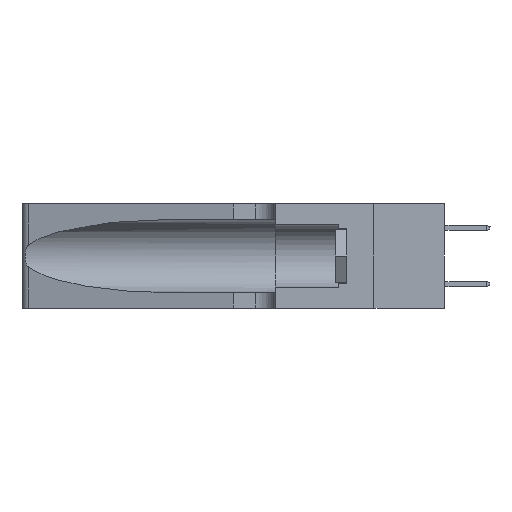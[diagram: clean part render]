
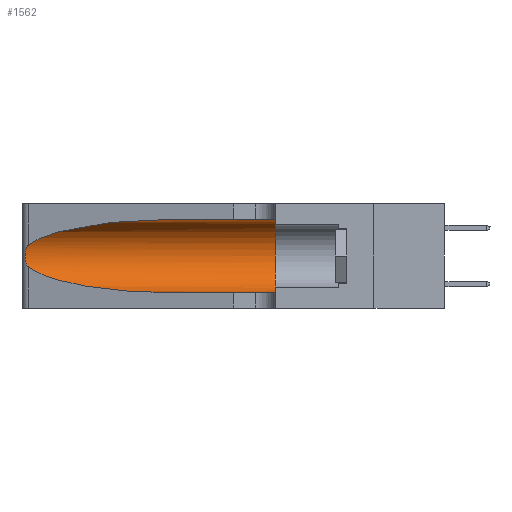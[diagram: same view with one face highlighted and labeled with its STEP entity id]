
A CAD part, left-side view. The second image highlights one B-rep face of the part: STEP entity #1562.
In plain terms, the highlighted cylindrical face has radius 3.308 mm (diameter 6.617 mm), a partial arc.
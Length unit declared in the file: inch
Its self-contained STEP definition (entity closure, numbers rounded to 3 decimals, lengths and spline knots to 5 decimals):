
#777 = CARTESIAN_POINT ( 'NONE',  ( 0.1305, 0.35, 0.05475 ) ) ;
#1447 = VERTEX_POINT ( 'NONE', #21464 ) ;
#1562 = ADVANCED_FACE ( 'NONE', ( #16014 ), #16576, .F. ) ;
#1746 = CARTESIAN_POINT ( 'NONE',  ( 0.25555, 1.22993, 0.14849 ) ) ;
#1816 = CARTESIAN_POINT ( 'NONE',  ( 0.25555, 1.22994, 0.2215 ) ) ;
#1904 = CARTESIAN_POINT ( 'NONE',  ( 0.1305, 0.72297, 0.31525 ) ) ;
#1925 =( BOUNDED_CURVE ( )  B_SPLINE_CURVE ( 3, ( #1904, #7684, #22179, #14631 ),
 .UNSPECIFIED., .F., .T. ) 
 B_SPLINE_CURVE_WITH_KNOTS ( ( 4, 4 ),
 ( 1.5708, 2.84003 ),
 .UNSPECIFIED. ) 
 CURVE ( )  GEOMETRIC_REPRESENTATION_ITEM ( )  RATIONAL_B_SPLINE_CURVE ( ( 1., 0.87, 0.87, 1. ) ) 
 REPRESENTATION_ITEM ( '' )  );
#1974 = CARTESIAN_POINT ( 'NONE',  ( 0.25639, 1.23186, 0.15144 ) ) ;
#1976 = DIRECTION ( 'NONE',  ( 0., -1., 0. ) ) ;
#2594 = VECTOR ( 'NONE', #1976, 39.37008 ) ;
#2981 = EDGE_CURVE ( 'NONE', #1447, #3437, #1925, .T. ) ;
#3400 =( BOUNDED_CURVE ( )  B_SPLINE_CURVE ( 3, ( #15521, #17353, #19363, #17596 ),
 .UNSPECIFIED., .F., .F. ) 
 B_SPLINE_CURVE_WITH_KNOTS ( ( 4, 4 ),
 ( 3.44316, 4.71239 ),
 .UNSPECIFIED. ) 
 CURVE ( )  GEOMETRIC_REPRESENTATION_ITEM ( )  RATIONAL_B_SPLINE_CURVE ( ( 1., 0.87, 0.87, 1. ) ) 
 REPRESENTATION_ITEM ( '' )  );
#3437 = VERTEX_POINT ( 'NONE', #15281 ) ;
#3655 = CARTESIAN_POINT ( 'NONE',  ( 0.25789, 1.23486, 0.15765 ) ) ;
#3808 = CARTESIAN_POINT ( 'NONE',  ( 0.25856, 1.23593, 0.16098 ) ) ;
#5525 = CARTESIAN_POINT ( 'NONE',  ( 0.25487, 1.22718, 0.14631 ) ) ;
#5551 = ORIENTED_EDGE ( 'NONE', *, *, #2981, .T. ) ;
#7432 = CARTESIAN_POINT ( 'NONE',  ( 0.25787, 1.23484, 0.2124 ) ) ;
#7684 = CARTESIAN_POINT ( 'NONE',  ( 0.18966, 0.96281, 0.31525 ) ) ;
#8034 = ORIENTED_EDGE ( 'NONE', *, *, #16308, .F. ) ;
#8298 = VERTEX_POINT ( 'NONE', #777 ) ;
#8983 = DIRECTION ( 'NONE',  ( 0., -1., 0. ) ) ;
#9079 = VERTEX_POINT ( 'NONE', #19063 ) ;
#9778 = EDGE_CURVE ( 'NONE', #20274, #8298, #18241, .T. ) ;
#9881 = DIRECTION ( 'NONE',  ( 0., 0., 1. ) ) ;
#10860 = CARTESIAN_POINT ( 'NONE',  ( 0.26018, 1.23835, 0.19895 ) ) ;
#10880 = CARTESIAN_POINT ( 'NONE',  ( 0.1305, 1.61858, 0.185 ) ) ;
#11398 = VERTEX_POINT ( 'NONE', #16741 ) ;
#11605 = CARTESIAN_POINT ( 'NONE',  ( 0.1305, 0.35, 0.185 ) ) ;
#12122 = EDGE_LOOP ( 'NONE', ( #5551, #12474, #19953, #23335, #19078, #8034 ) ) ;
#12474 = ORIENTED_EDGE ( 'NONE', *, *, #21855, .T. ) ;
#12660 = AXIS2_PLACEMENT_3D ( 'NONE', #11605, #20731, #9881 ) ;
#12752 = CARTESIAN_POINT ( 'NONE',  ( 0.25639, 1.23184, 0.21858 ) ) ;
#12831 = CARTESIAN_POINT ( 'NONE',  ( 0.26075, 1.23896, 0.178 ) ) ;
#12861 = LINE ( 'NONE', #14943, #2594 ) ;
#12899 = CARTESIAN_POINT ( 'NONE',  ( 0.25487, 1.22718, 0.22369 ) ) ;
#14551 = CARTESIAN_POINT ( 'NONE',  ( 0.25854, 1.2359, 0.20912 ) ) ;
#14631 = CARTESIAN_POINT ( 'NONE',  ( 0.25487, 1.22718, 0.22369 ) ) ;
#14943 = CARTESIAN_POINT ( 'NONE',  ( 0.1305, 1.61858, 0.31525 ) ) ;
#15281 = CARTESIAN_POINT ( 'NONE',  ( 0.25487, 1.22718, 0.22369 ) ) ;
#15355 = CARTESIAN_POINT ( 'NONE',  ( 0.26017, 1.23833, 0.17102 ) ) ;
#15521 = CARTESIAN_POINT ( 'NONE',  ( 0.25487, 1.22718, 0.14631 ) ) ;
#16014 = FACE_OUTER_BOUND ( 'NONE', #12122, .T. ) ;
#16308 = EDGE_CURVE ( 'NONE', #1447, #20274, #12861, .T. ) ;
#16330 = VECTOR ( 'NONE', #20037, 39.37008 ) ;
#16576 = CYLINDRICAL_SURFACE ( 'NONE', #19695, 0.13025 ) ;
#16591 = CARTESIAN_POINT ( 'NONE',  ( 0.1305, 1.61858, 0.05475 ) ) ;
#16741 = CARTESIAN_POINT ( 'NONE',  ( 0.1305, 0.72297, 0.05475 ) ) ;
#17353 = CARTESIAN_POINT ( 'NONE',  ( 0.2373, 1.15595, 0.08982 ) ) ;
#17596 = CARTESIAN_POINT ( 'NONE',  ( 0.1305, 0.72297, 0.05475 ) ) ;
#18066 = CARTESIAN_POINT ( 'NONE',  ( 0.26075, 1.23896, 0.19203 ) ) ;
#18241 = CIRCLE ( 'NONE', #12660, 0.13025 ) ;
#18502 = EDGE_CURVE ( 'NONE', #9079, #11398, #3400, .T. ) ;
#19063 = CARTESIAN_POINT ( 'NONE',  ( 0.25487, 1.22718, 0.14631 ) ) ;
#19078 = ORIENTED_EDGE ( 'NONE', *, *, #9778, .F. ) ;
#19363 = CARTESIAN_POINT ( 'NONE',  ( 0.18966, 0.96281, 0.05475 ) ) ;
#19695 = AXIS2_PLACEMENT_3D ( 'NONE', #10880, #8983, #21654 ) ;
#19953 = ORIENTED_EDGE ( 'NONE', *, *, #18502, .T. ) ;
#20037 = DIRECTION ( 'NONE',  ( 0., -1., 0. ) ) ;
#20274 = VERTEX_POINT ( 'NONE', #21312 ) ;
#20325 = LINE ( 'NONE', #16591, #16330 ) ;
#20731 = DIRECTION ( 'NONE',  ( 0., 1., 0. ) ) ;
#21312 = CARTESIAN_POINT ( 'NONE',  ( 0.1305, 0.35, 0.31525 ) ) ;
#21464 = CARTESIAN_POINT ( 'NONE',  ( 0.1305, 0.72297, 0.31525 ) ) ;
#21654 = DIRECTION ( 'NONE',  ( 0., 0., -1. ) ) ;
#21855 = EDGE_CURVE ( 'NONE', #3437, #9079, #23366, .T. ) ;
#22179 = CARTESIAN_POINT ( 'NONE',  ( 0.2373, 1.15595, 0.28018 ) ) ;
#22340 = EDGE_CURVE ( 'NONE', #11398, #8298, #20325, .T. ) ;
#23335 = ORIENTED_EDGE ( 'NONE', *, *, #22340, .T. ) ;
#23366 = B_SPLINE_CURVE_WITH_KNOTS ( 'NONE', 3,
 ( #12899, #1816, #12752, #7432, #14551, #10860, #18066, #12831, #15355, #3808, #3655, #1974, #1746, #5525 ),
 .UNSPECIFIED., .F., .F.,
 ( 4, 2, 2, 2, 2, 2, 4 ),
 ( 0., 0.00027, 0.00053, 0.00107, 0.0016, 0.00187, 0.00214 ),
 .UNSPECIFIED. ) ;
